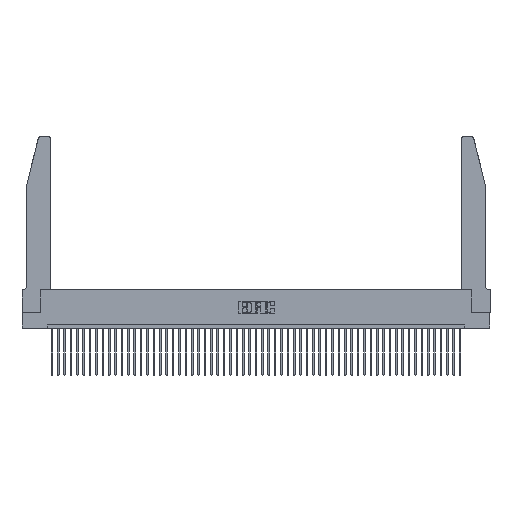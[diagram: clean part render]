
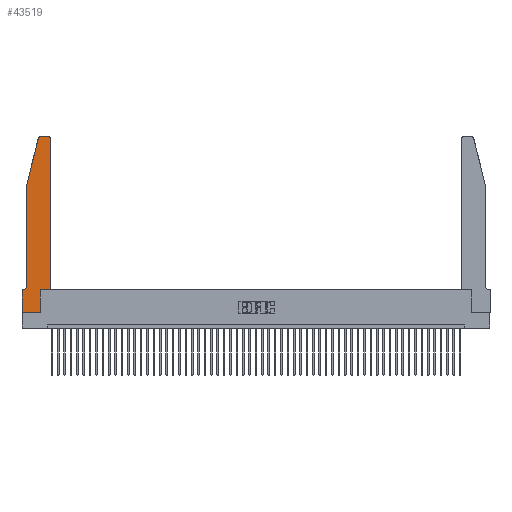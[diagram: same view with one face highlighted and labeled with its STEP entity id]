
A CAD part, top view. The second image highlights one B-rep face of the part: STEP entity #43519.
In plain terms, the highlighted planar face has unit normal (0, 0, 1).
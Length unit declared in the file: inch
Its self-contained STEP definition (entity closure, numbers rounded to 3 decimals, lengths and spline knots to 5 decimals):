
#360 = VERTEX_POINT ( 'NONE', #6816 ) ;
#769 = CARTESIAN_POINT ( 'NONE',  ( 0.4505, 0.35, 0.37 ) ) ;
#834 = VERTEX_POINT ( 'NONE', #15551 ) ;
#848 = CARTESIAN_POINT ( 'NONE',  ( 0.0755, 2., 0.37 ) ) ;
#1139 = EDGE_CURVE ( 'NONE', #17432, #16469, #15703, .T. ) ;
#1536 = VERTEX_POINT ( 'NONE', #769 ) ;
#1564 = CARTESIAN_POINT ( 'NONE',  ( 0.2605, 2.75, 0.37 ) ) ;
#2244 = DIRECTION ( 'NONE',  ( -1., 0., 0. ) ) ;
#2598 = ORIENTED_EDGE ( 'NONE', *, *, #33289, .T. ) ;
#3294 = DIRECTION ( 'NONE',  ( 0., 0., 1. ) ) ;
#3797 = ORIENTED_EDGE ( 'NONE', *, *, #32555, .T. ) ;
#4083 = AXIS2_PLACEMENT_3D ( 'NONE', #26392, #26737, #11093 ) ;
#4134 = VECTOR ( 'NONE', #26177, 39.37008 ) ;
#4694 = CARTESIAN_POINT ( 'NONE',  ( 0., 0., 0.37 ) ) ;
#5781 = CARTESIAN_POINT ( 'NONE',  ( 0.4505, 0.35, 0.37 ) ) ;
#6816 = CARTESIAN_POINT ( 'NONE',  ( 0.2865, 0., 0.37 ) ) ;
#7394 = CARTESIAN_POINT ( 'NONE',  ( 0.284, 2.72, 0.37 ) ) ;
#7792 = CARTESIAN_POINT ( 'NONE',  ( 0.4205, 2.72, 0.37 ) ) ;
#7955 = DIRECTION ( 'NONE',  ( 1., 0., 0. ) ) ;
#8109 = VECTOR ( 'NONE', #30694, 39.37008 ) ;
#9708 = CARTESIAN_POINT ( 'NONE',  ( 0., 0.35, 0.37 ) ) ;
#10321 = DIRECTION ( 'NONE',  ( 1., 0., 0. ) ) ;
#10346 = ORIENTED_EDGE ( 'NONE', *, *, #46516, .T. ) ;
#11093 = DIRECTION ( 'NONE',  ( -1., 0., 0. ) ) ;
#11310 = ORIENTED_EDGE ( 'NONE', *, *, #39325, .T. ) ;
#12477 = VERTEX_POINT ( 'NONE', #17417 ) ;
#12806 = DIRECTION ( 'NONE',  ( 0., 1., 0. ) ) ;
#13097 = ORIENTED_EDGE ( 'NONE', *, *, #28617, .T. ) ;
#14485 = CARTESIAN_POINT ( 'NONE',  ( 0.2865, 0.35, 0.37 ) ) ;
#14653 = ORIENTED_EDGE ( 'NONE', *, *, #24473, .T. ) ;
#14782 = LINE ( 'NONE', #1564, #40558 ) ;
#15551 = CARTESIAN_POINT ( 'NONE',  ( 0.0755, 0.42, 0.37 ) ) ;
#15703 = LINE ( 'NONE', #18815, #4134 ) ;
#16452 = VERTEX_POINT ( 'NONE', #35984 ) ;
#16469 = VERTEX_POINT ( 'NONE', #4694 ) ;
#16989 = CARTESIAN_POINT ( 'NONE',  ( 0.0755, 0.35, 0.37 ) ) ;
#17417 = CARTESIAN_POINT ( 'NONE',  ( 0.25487, 2.72718, 0.37 ) ) ;
#17432 = VERTEX_POINT ( 'NONE', #9708 ) ;
#18015 = LINE ( 'NONE', #32157, #48025 ) ;
#18134 = CARTESIAN_POINT ( 'NONE',  ( 0.4205, 2.75, 0.37 ) ) ;
#18491 = CARTESIAN_POINT ( 'NONE',  ( 0.284, 2.75, 0.37 ) ) ;
#18578 = EDGE_CURVE ( 'NONE', #49937, #12477, #37839, .T. ) ;
#18815 = CARTESIAN_POINT ( 'NONE',  ( 0., 0., 0.37 ) ) ;
#19404 = EDGE_CURVE ( 'NONE', #834, #42028, #43266, .T. ) ;
#21673 = CARTESIAN_POINT ( 'NONE',  ( 0.4505, 0.35, 0.37 ) ) ;
#23336 = DIRECTION ( 'NONE',  ( 1., 0., 0. ) ) ;
#24473 = EDGE_CURVE ( 'NONE', #1536, #16452, #49396, .T. ) ;
#26177 = DIRECTION ( 'NONE',  ( 0., -1., 0. ) ) ;
#26392 = CARTESIAN_POINT ( 'NONE',  ( 0.0055, 0.42, 0.37 ) ) ;
#26406 = PLANE ( 'NONE',  #43327 ) ;
#26493 = EDGE_CURVE ( 'NONE', #16452, #42332, #38350, .T. ) ;
#26645 = ORIENTED_EDGE ( 'NONE', *, *, #19404, .T. ) ;
#26737 = DIRECTION ( 'NONE',  ( 0., 0., -1. ) ) ;
#26904 = VECTOR ( 'NONE', #10321, 39.37008 ) ;
#26913 = VERTEX_POINT ( 'NONE', #47395 ) ;
#27529 = DIRECTION ( 'NONE',  ( 0., 0., 1. ) ) ;
#27605 = DIRECTION ( 'NONE',  ( 0., -1., 0. ) ) ;
#27734 = VECTOR ( 'NONE', #33270, 39.37008 ) ;
#28617 = EDGE_CURVE ( 'NONE', #12477, #33893, #36855, .T. ) ;
#30694 = DIRECTION ( 'NONE',  ( -0.239, -0.971, 0. ) ) ;
#31258 = LINE ( 'NONE', #14485, #42933 ) ;
#31833 = ORIENTED_EDGE ( 'NONE', *, *, #49606, .T. ) ;
#31875 = CARTESIAN_POINT ( 'NONE',  ( 0.0055, 0.35, 0.37 ) ) ;
#32157 = CARTESIAN_POINT ( 'NONE',  ( 0., 0., 0.37 ) ) ;
#32555 = EDGE_CURVE ( 'NONE', #16469, #360, #18015, .T. ) ;
#33270 = DIRECTION ( 'NONE',  ( -1., 0., 0. ) ) ;
#33289 = EDGE_CURVE ( 'NONE', #42028, #17432, #49773, .T. ) ;
#33313 = DIRECTION ( 'NONE',  ( 0., 1., 0. ) ) ;
#33893 = VERTEX_POINT ( 'NONE', #848 ) ;
#34738 = EDGE_CURVE ( 'NONE', #26913, #1536, #48361, .T. ) ;
#35006 = CARTESIAN_POINT ( 'NONE',  ( 0.0755, 2., 0.37 ) ) ;
#35146 = AXIS2_PLACEMENT_3D ( 'NONE', #7394, #3294, #38874 ) ;
#35795 = EDGE_LOOP ( 'NONE', ( #10346, #50293, #13097, #31833, #26645, #2598, #36924, #3797, #11310, #49377, #14653, #39515 ) ) ;
#35954 = DIRECTION ( 'NONE',  ( 1., 0., 0. ) ) ;
#35984 = CARTESIAN_POINT ( 'NONE',  ( 0.4505, 2.72, 0.37 ) ) ;
#36855 = LINE ( 'NONE', #35006, #8109 ) ;
#36924 = ORIENTED_EDGE ( 'NONE', *, *, #1139, .T. ) ;
#37839 = CIRCLE ( 'NONE', #35146, 0.03 ) ;
#38350 = CIRCLE ( 'NONE', #45848, 0.03 ) ;
#38874 = DIRECTION ( 'NONE',  ( 1., 0., 0. ) ) ;
#39190 = VECTOR ( 'NONE', #27605, 39.37008 ) ;
#39325 = EDGE_CURVE ( 'NONE', #360, #26913, #31258, .T. ) ;
#39331 = CARTESIAN_POINT ( 'NONE',  ( 0.0755, 2., 0.37 ) ) ;
#39515 = ORIENTED_EDGE ( 'NONE', *, *, #26493, .T. ) ;
#40558 = VECTOR ( 'NONE', #2244, 39.37008 ) ;
#42028 = VERTEX_POINT ( 'NONE', #31875 ) ;
#42332 = VERTEX_POINT ( 'NONE', #18134 ) ;
#42933 = VECTOR ( 'NONE', #33313, 39.37008 ) ;
#43266 = CIRCLE ( 'NONE', #4083, 0.07 ) ;
#43327 = AXIS2_PLACEMENT_3D ( 'NONE', #50021, #50541, #23336 ) ;
#43442 = LINE ( 'NONE', #39331, #39190 ) ;
#43519 = ADVANCED_FACE ( 'NONE', ( #44552 ), #26406, .T. ) ;
#44552 = FACE_OUTER_BOUND ( 'NONE', #35795, .T. ) ;
#45774 = VECTOR ( 'NONE', #12806, 39.37008 ) ;
#45848 = AXIS2_PLACEMENT_3D ( 'NONE', #7792, #27529, #7955 ) ;
#46516 = EDGE_CURVE ( 'NONE', #42332, #49937, #14782, .T. ) ;
#47395 = CARTESIAN_POINT ( 'NONE',  ( 0.2865, 0.35, 0.37 ) ) ;
#48025 = VECTOR ( 'NONE', #35954, 39.37008 ) ;
#48361 = LINE ( 'NONE', #21673, #26904 ) ;
#49377 = ORIENTED_EDGE ( 'NONE', *, *, #34738, .T. ) ;
#49396 = LINE ( 'NONE', #5781, #45774 ) ;
#49606 = EDGE_CURVE ( 'NONE', #33893, #834, #43442, .T. ) ;
#49773 = LINE ( 'NONE', #16989, #27734 ) ;
#49937 = VERTEX_POINT ( 'NONE', #18491 ) ;
#50021 = CARTESIAN_POINT ( 'NONE',  ( 0., 0.35, 0.37 ) ) ;
#50293 = ORIENTED_EDGE ( 'NONE', *, *, #18578, .T. ) ;
#50541 = DIRECTION ( 'NONE',  ( 0., 0., 1. ) ) ;
